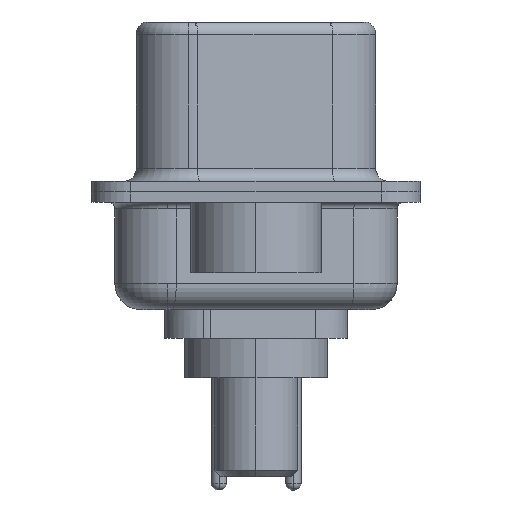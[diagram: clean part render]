
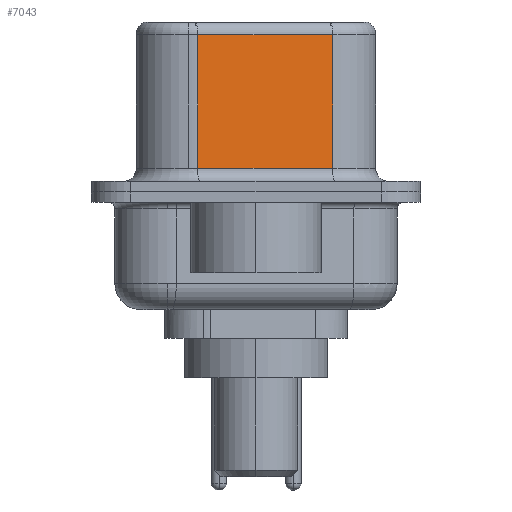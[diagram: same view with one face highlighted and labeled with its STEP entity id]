
A CAD part, left-side view. The second image highlights one B-rep face of the part: STEP entity #7043.
In plain terms, the highlighted planar face has unit normal (-0.985, -0.174, 0).
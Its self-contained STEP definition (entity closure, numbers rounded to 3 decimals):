
#260 = DIRECTION ( 'NONE',  ( -0.174, 0.985, 0. ) ) ;
#289 = CARTESIAN_POINT ( 'NONE',  ( 3.67, 2.233, 6.52 ) ) ;
#1632 = VECTOR ( 'NONE', #5458, 1000. ) ;
#1652 = LINE ( 'NONE', #289, #15525 ) ;
#1816 = VECTOR ( 'NONE', #2929, 1000. ) ;
#2250 = CARTESIAN_POINT ( 'NONE',  ( 4.58, -2.927, 6.02 ) ) ;
#2693 = ORIENTED_EDGE ( 'NONE', *, *, #14323, .T. ) ;
#2929 = DIRECTION ( 'NONE',  ( 0.174, -0.985, 0. ) ) ;
#3014 = FACE_OUTER_BOUND ( 'NONE', #5612, .T. ) ;
#3469 = ORIENTED_EDGE ( 'NONE', *, *, #14778, .F. ) ;
#4290 = CARTESIAN_POINT ( 'NONE',  ( 4.58, -2.927, 0.9 ) ) ;
#4767 = LINE ( 'NONE', #21735, #13762 ) ;
#5458 = DIRECTION ( 'NONE',  ( 0., 0., -1. ) ) ;
#5612 = EDGE_LOOP ( 'NONE', ( #3469, #20107, #2693, #17407 ) ) ;
#6586 = LINE ( 'NONE', #10814, #1632 ) ;
#6968 = VERTEX_POINT ( 'NONE', #4290 ) ;
#7043 = ADVANCED_FACE ( 'NONE', ( #3014 ), #17826, .F. ) ;
#7355 = LINE ( 'NONE', #23166, #1816 ) ;
#7827 = EDGE_CURVE ( 'NONE', #13033, #6968, #7355, .T. ) ;
#8947 = AXIS2_PLACEMENT_3D ( 'NONE', #19150, #18313, #17562 ) ;
#10189 = EDGE_CURVE ( 'NONE', #12126, #10870, #4767, .T. ) ;
#10814 = CARTESIAN_POINT ( 'NONE',  ( 4.58, -2.927, 6.52 ) ) ;
#10870 = VERTEX_POINT ( 'NONE', #16842 ) ;
#12126 = VERTEX_POINT ( 'NONE', #2250 ) ;
#13033 = VERTEX_POINT ( 'NONE', #17917 ) ;
#13762 = VECTOR ( 'NONE', #260, 1000. ) ;
#14323 = EDGE_CURVE ( 'NONE', #10870, #13033, #1652, .T. ) ;
#14778 = EDGE_CURVE ( 'NONE', #12126, #6968, #6586, .T. ) ;
#15525 = VECTOR ( 'NONE', #21759, 1000. ) ;
#16842 = CARTESIAN_POINT ( 'NONE',  ( 3.67, 2.233, 6.02 ) ) ;
#17407 = ORIENTED_EDGE ( 'NONE', *, *, #7827, .T. ) ;
#17562 = DIRECTION ( 'NONE',  ( -0.174, 0.985, 0. ) ) ;
#17826 = PLANE ( 'NONE',  #8947 ) ;
#17917 = CARTESIAN_POINT ( 'NONE',  ( 3.67, 2.233, 0.9 ) ) ;
#18313 = DIRECTION ( 'NONE',  ( 0.985, 0.174, 0. ) ) ;
#19150 = CARTESIAN_POINT ( 'NONE',  ( 4.58, -2.927, 6.52 ) ) ;
#20107 = ORIENTED_EDGE ( 'NONE', *, *, #10189, .T. ) ;
#21735 = CARTESIAN_POINT ( 'NONE',  ( 4.58, -2.927, 6.02 ) ) ;
#21759 = DIRECTION ( 'NONE',  ( 0., 0., -1. ) ) ;
#23166 = CARTESIAN_POINT ( 'NONE',  ( 4.58, -2.927, 0.9 ) ) ;
